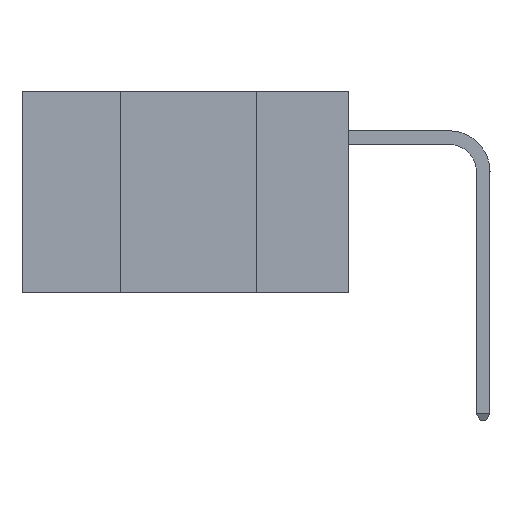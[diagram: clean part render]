
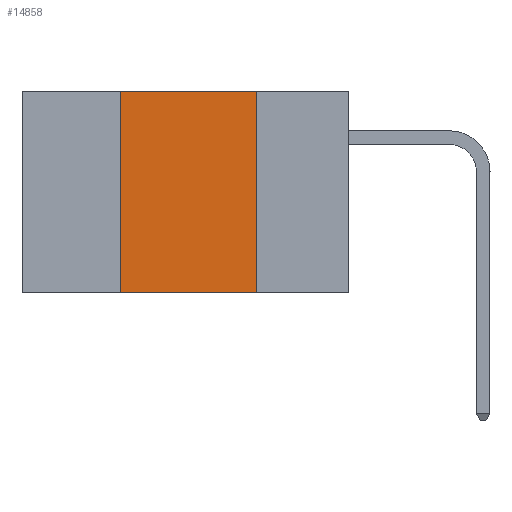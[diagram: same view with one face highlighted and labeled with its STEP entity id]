
A CAD part, left-side view. The second image highlights one B-rep face of the part: STEP entity #14858.
In plain terms, the highlighted planar face has unit normal (-1, 0, 0).
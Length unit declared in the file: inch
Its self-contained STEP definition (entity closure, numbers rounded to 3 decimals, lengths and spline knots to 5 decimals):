
#2353 = LINE ( 'NONE', #36570, #12045 ) ;
#3126 = CARTESIAN_POINT ( 'NONE',  ( 0., 0.17, -0.37 ) ) ;
#3308 = CARTESIAN_POINT ( 'NONE',  ( 0., 0.6, 0. ) ) ;
#4690 = CARTESIAN_POINT ( 'NONE',  ( 0., 0.42, -0.37 ) ) ;
#8115 = EDGE_CURVE ( 'NONE', #33679, #9402, #29415, .T. ) ;
#9402 = VERTEX_POINT ( 'NONE', #3126 ) ;
#10749 = LINE ( 'NONE', #27236, #14861 ) ;
#10781 = ORIENTED_EDGE ( 'NONE', *, *, #21224, .F. ) ;
#10898 = CARTESIAN_POINT ( 'NONE',  ( 0., 0.17, 0. ) ) ;
#11507 = VERTEX_POINT ( 'NONE', #4690 ) ;
#11776 = CARTESIAN_POINT ( 'NONE',  ( 0., 0.6, 0. ) ) ;
#12030 = VECTOR ( 'NONE', #26896, 39.37008 ) ;
#12045 = VECTOR ( 'NONE', #16891, 39.37008 ) ;
#12858 = ORIENTED_EDGE ( 'NONE', *, *, #36433, .F. ) ;
#13572 = EDGE_CURVE ( 'NONE', #11507, #9402, #2353, .T. ) ;
#14858 = ADVANCED_FACE ( 'NONE', ( #30856 ), #16111, .F. ) ;
#14861 = VECTOR ( 'NONE', #23641, 39.37008 ) ;
#16111 = PLANE ( 'NONE',  #37075 ) ;
#16352 = ORIENTED_EDGE ( 'NONE', *, *, #8115, .F. ) ;
#16891 = DIRECTION ( 'NONE',  ( 0., -1., 0. ) ) ;
#19773 = DIRECTION ( 'NONE',  ( 1., 0., 0. ) ) ;
#21224 = EDGE_CURVE ( 'NONE', #42108, #33679, #40883, .T. ) ;
#21678 = CARTESIAN_POINT ( 'NONE',  ( 0., 0.17, 0. ) ) ;
#21975 = EDGE_LOOP ( 'NONE', ( #16352, #10781, #12858, #24242 ) ) ;
#23641 = DIRECTION ( 'NONE',  ( 0., 0., 1. ) ) ;
#24242 = ORIENTED_EDGE ( 'NONE', *, *, #13572, .T. ) ;
#24608 = DIRECTION ( 'NONE',  ( 0., -1., 0. ) ) ;
#26127 = DIRECTION ( 'NONE',  ( 0., 0., -1. ) ) ;
#26896 = DIRECTION ( 'NONE',  ( 0., 0., -1. ) ) ;
#27236 = CARTESIAN_POINT ( 'NONE',  ( 0., 0.42, 0. ) ) ;
#28726 = CARTESIAN_POINT ( 'NONE',  ( 0., 0.42, 0. ) ) ;
#29415 = LINE ( 'NONE', #10898, #12030 ) ;
#30856 = FACE_OUTER_BOUND ( 'NONE', #21975, .T. ) ;
#33679 = VERTEX_POINT ( 'NONE', #21678 ) ;
#36433 = EDGE_CURVE ( 'NONE', #11507, #42108, #10749, .T. ) ;
#36570 = CARTESIAN_POINT ( 'NONE',  ( 0., 0.6, -0.37 ) ) ;
#37075 = AXIS2_PLACEMENT_3D ( 'NONE', #3308, #19773, #26127 ) ;
#39819 = VECTOR ( 'NONE', #24608, 39.37008 ) ;
#40883 = LINE ( 'NONE', #11776, #39819 ) ;
#42108 = VERTEX_POINT ( 'NONE', #28726 ) ;
